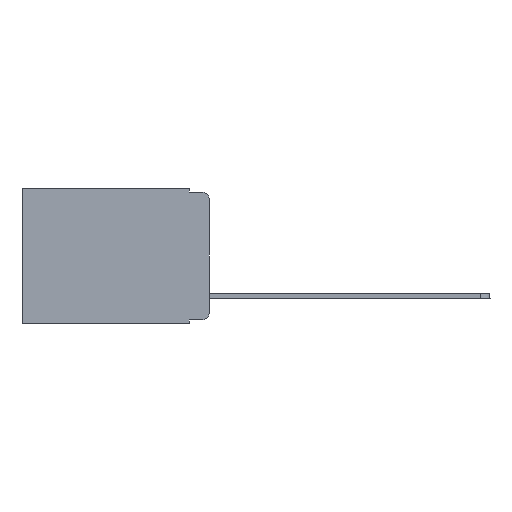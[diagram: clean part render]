
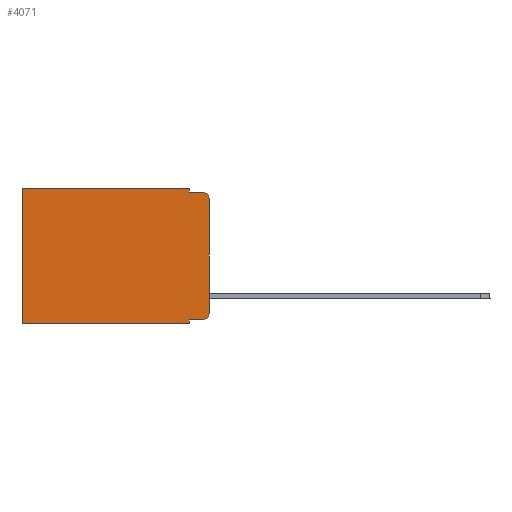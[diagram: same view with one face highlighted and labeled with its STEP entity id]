
A CAD part, left-side view. The second image highlights one B-rep face of the part: STEP entity #4071.
In plain terms, the highlighted planar face has unit normal (-1, 0, 0).
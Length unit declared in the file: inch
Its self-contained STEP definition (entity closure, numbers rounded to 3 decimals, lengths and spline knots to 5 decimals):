
#70 = ORIENTED_EDGE ( 'NONE', *, *, #16366, .F. ) ;
#149 = CARTESIAN_POINT ( 'NONE',  ( 0.298, 0.473, 0. ) ) ;
#152 = CARTESIAN_POINT ( 'NONE',  ( 0.298, 0.051, 0. ) ) ;
#575 = CARTESIAN_POINT ( 'NONE',  ( 0.298, 0., -0.313 ) ) ;
#750 = VERTEX_POINT ( 'NONE', #3914 ) ;
#1035 = DIRECTION ( 'NONE',  ( -1., 0., 0. ) ) ;
#1239 = EDGE_CURVE ( 'NONE', #15717, #10991, #4442, .T. ) ;
#2059 = CARTESIAN_POINT ( 'NONE',  ( 0.298, 0.051, 0. ) ) ;
#2480 = CARTESIAN_POINT ( 'NONE',  ( 0.298, 0.051, -0.01 ) ) ;
#2867 = VECTOR ( 'NONE', #5871, 39.37008 ) ;
#2929 = CIRCLE ( 'NONE', #3472, 0.02 ) ;
#3049 = AXIS2_PLACEMENT_3D ( 'NONE', #18022, #7928, #16417 ) ;
#3218 = VECTOR ( 'NONE', #11085, 39.37008 ) ;
#3472 = AXIS2_PLACEMENT_3D ( 'NONE', #16839, #6802, #10157 ) ;
#3799 = AXIS2_PLACEMENT_3D ( 'NONE', #12991, #1035, #16230 ) ;
#3914 = CARTESIAN_POINT ( 'NONE',  ( 0.298, 0.051, -0.01 ) ) ;
#4071 = ADVANCED_FACE ( 'NONE', ( #5344 ), #11267, .F. ) ;
#4121 = CARTESIAN_POINT ( 'NONE',  ( 0.298, 0., -0.03 ) ) ;
#4259 = ORIENTED_EDGE ( 'NONE', *, *, #10318, .T. ) ;
#4442 = LINE ( 'NONE', #9376, #2867 ) ;
#5137 = CARTESIAN_POINT ( 'NONE',  ( 0.298, 0.473, -0.343 ) ) ;
#5163 = DIRECTION ( 'NONE',  ( 0., 0., -1. ) ) ;
#5289 = VERTEX_POINT ( 'NONE', #4121 ) ;
#5344 = FACE_OUTER_BOUND ( 'NONE', #11980, .T. ) ;
#5650 = LINE ( 'NONE', #12686, #18493 ) ;
#5871 = DIRECTION ( 'NONE',  ( 0., 1., 0. ) ) ;
#6187 = DIRECTION ( 'NONE',  ( 0., -1., 0. ) ) ;
#6494 = ORIENTED_EDGE ( 'NONE', *, *, #14451, .F. ) ;
#6587 = CARTESIAN_POINT ( 'NONE',  ( 0.298, 0.051, 0. ) ) ;
#6802 = DIRECTION ( 'NONE',  ( -1., 0., 0. ) ) ;
#6885 = ORIENTED_EDGE ( 'NONE', *, *, #1239, .F. ) ;
#7062 = EDGE_CURVE ( 'NONE', #5289, #13746, #18429, .T. ) ;
#7541 = VECTOR ( 'NONE', #5163, 39.37008 ) ;
#7928 = DIRECTION ( 'NONE',  ( 1., 0., 0. ) ) ;
#7951 = ORIENTED_EDGE ( 'NONE', *, *, #16755, .T. ) ;
#8036 = CARTESIAN_POINT ( 'NONE',  ( 0.298, 0., 0. ) ) ;
#8616 = EDGE_CURVE ( 'NONE', #18689, #15717, #17031, .T. ) ;
#9376 = CARTESIAN_POINT ( 'NONE',  ( 0.298, 0., -0.343 ) ) ;
#9496 = VECTOR ( 'NONE', #14554, 39.37008 ) ;
#9529 = CARTESIAN_POINT ( 'NONE',  ( 0.298, 0.473, 0. ) ) ;
#9622 = LINE ( 'NONE', #149, #7541 ) ;
#9744 = LINE ( 'NONE', #12860, #9496 ) ;
#10157 = DIRECTION ( 'NONE',  ( 0., 0., -1. ) ) ;
#10318 = EDGE_CURVE ( 'NONE', #15556, #10991, #9622, .T. ) ;
#10505 = DIRECTION ( 'NONE',  ( 0., 0., -1. ) ) ;
#10596 = ORIENTED_EDGE ( 'NONE', *, *, #18865, .T. ) ;
#10991 = VERTEX_POINT ( 'NONE', #5137 ) ;
#11085 = DIRECTION ( 'NONE',  ( 0., 1., 0. ) ) ;
#11267 = PLANE ( 'NONE',  #3049 ) ;
#11980 = EDGE_LOOP ( 'NONE', ( #70, #21578, #6494, #16833, #20627, #4259, #6885, #13574, #10596, #7951 ) ) ;
#12126 = DIRECTION ( 'NONE',  ( 0., 0., -1. ) ) ;
#12686 = CARTESIAN_POINT ( 'NONE',  ( 0.298, 0.051, -0.333 ) ) ;
#12860 = CARTESIAN_POINT ( 'NONE',  ( 0.298, 0., 0. ) ) ;
#12991 = CARTESIAN_POINT ( 'NONE',  ( 0.298, 0.02, -0.03 ) ) ;
#13276 = VERTEX_POINT ( 'NONE', #15843 ) ;
#13574 = ORIENTED_EDGE ( 'NONE', *, *, #8616, .F. ) ;
#13746 = VERTEX_POINT ( 'NONE', #16115 ) ;
#13975 = VERTEX_POINT ( 'NONE', #2059 ) ;
#14451 = EDGE_CURVE ( 'NONE', #750, #13746, #18709, .T. ) ;
#14554 = DIRECTION ( 'NONE',  ( 0., 0., -1. ) ) ;
#14959 = CARTESIAN_POINT ( 'NONE',  ( 0.298, 0.051, -0.343 ) ) ;
#15256 = VERTEX_POINT ( 'NONE', #575 ) ;
#15401 = EDGE_CURVE ( 'NONE', #13975, #15556, #21562, .T. ) ;
#15556 = VERTEX_POINT ( 'NONE', #9529 ) ;
#15717 = VERTEX_POINT ( 'NONE', #14959 ) ;
#15843 = CARTESIAN_POINT ( 'NONE',  ( 0.298, 0.02, -0.333 ) ) ;
#16115 = CARTESIAN_POINT ( 'NONE',  ( 0.298, 0.02, -0.01 ) ) ;
#16230 = DIRECTION ( 'NONE',  ( 0., 0., -1. ) ) ;
#16366 = EDGE_CURVE ( 'NONE', #5289, #15256, #9744, .T. ) ;
#16417 = DIRECTION ( 'NONE',  ( 0., 0., -1. ) ) ;
#16755 = EDGE_CURVE ( 'NONE', #13276, #15256, #2929, .T. ) ;
#16789 = VECTOR ( 'NONE', #10505, 39.37008 ) ;
#16833 = ORIENTED_EDGE ( 'NONE', *, *, #21279, .F. ) ;
#16839 = CARTESIAN_POINT ( 'NONE',  ( 0.298, 0.02, -0.313 ) ) ;
#17031 = LINE ( 'NONE', #6587, #16789 ) ;
#17340 = DIRECTION ( 'NONE',  ( 0., -1., 0. ) ) ;
#17826 = LINE ( 'NONE', #152, #20417 ) ;
#18022 = CARTESIAN_POINT ( 'NONE',  ( 0.298, 0., 0. ) ) ;
#18429 = CIRCLE ( 'NONE', #3799, 0.02 ) ;
#18493 = VECTOR ( 'NONE', #6187, 39.37008 ) ;
#18689 = VERTEX_POINT ( 'NONE', #19938 ) ;
#18709 = LINE ( 'NONE', #2480, #19760 ) ;
#18865 = EDGE_CURVE ( 'NONE', #18689, #13276, #5650, .T. ) ;
#19760 = VECTOR ( 'NONE', #17340, 39.37008 ) ;
#19938 = CARTESIAN_POINT ( 'NONE',  ( 0.298, 0.051, -0.333 ) ) ;
#20417 = VECTOR ( 'NONE', #12126, 39.37008 ) ;
#20627 = ORIENTED_EDGE ( 'NONE', *, *, #15401, .T. ) ;
#21279 = EDGE_CURVE ( 'NONE', #13975, #750, #17826, .T. ) ;
#21562 = LINE ( 'NONE', #8036, #3218 ) ;
#21578 = ORIENTED_EDGE ( 'NONE', *, *, #7062, .T. ) ;
